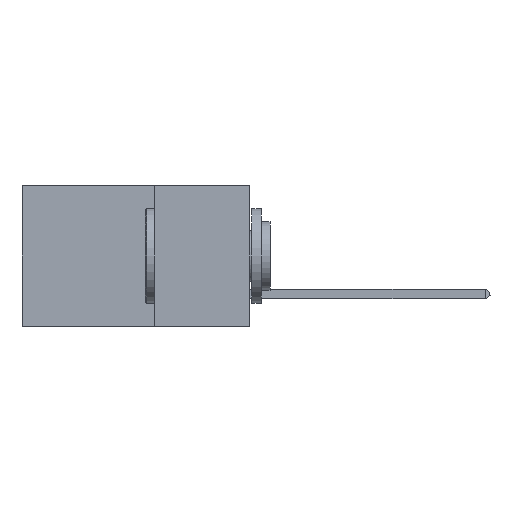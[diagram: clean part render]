
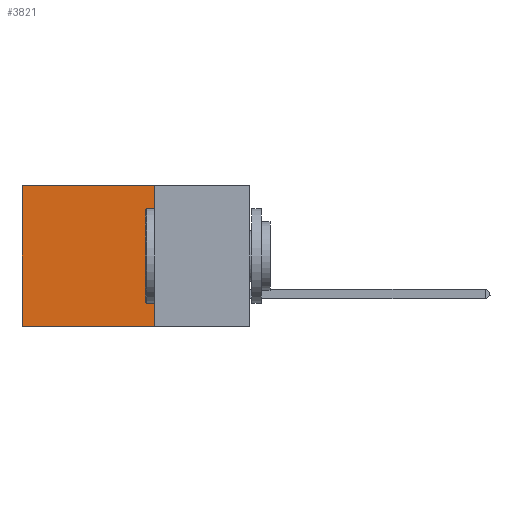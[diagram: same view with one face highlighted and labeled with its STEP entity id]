
A CAD part, left-side view. The second image highlights one B-rep face of the part: STEP entity #3821.
In plain terms, the highlighted planar face has unit normal (-1, 0, 0).
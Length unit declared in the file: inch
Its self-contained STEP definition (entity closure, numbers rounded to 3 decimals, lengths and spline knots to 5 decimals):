
#472 = CARTESIAN_POINT ( 'NONE',  ( 0.2875, 0.25, 0. ) ) ;
#618 = CARTESIAN_POINT ( 'NONE',  ( 0.2875, 0.6, -0.37 ) ) ;
#3821 = ADVANCED_FACE ( 'NONE', ( #30161 ), #40266, .F. ) ;
#4129 = LINE ( 'NONE', #29241, #27058 ) ;
#5090 = EDGE_LOOP ( 'NONE', ( #18821, #26132, #16756, #10674 ) ) ;
#5831 = CARTESIAN_POINT ( 'NONE',  ( 0.2875, 0.25, 0. ) ) ;
#8003 = LINE ( 'NONE', #39644, #36180 ) ;
#9676 = CARTESIAN_POINT ( 'NONE',  ( 0.2875, 0.25, 0. ) ) ;
#10134 = CARTESIAN_POINT ( 'NONE',  ( 0.2875, 0.25, 0. ) ) ;
#10674 = ORIENTED_EDGE ( 'NONE', *, *, #26300, .T. ) ;
#10934 = VERTEX_POINT ( 'NONE', #19697 ) ;
#12505 = EDGE_CURVE ( 'NONE', #19059, #10934, #37296, .T. ) ;
#12753 = EDGE_CURVE ( 'NONE', #10934, #43360, #8003, .T. ) ;
#14618 = EDGE_CURVE ( 'NONE', #18828, #43360, #4129, .T. ) ;
#16756 = ORIENTED_EDGE ( 'NONE', *, *, #12505, .F. ) ;
#18821 = ORIENTED_EDGE ( 'NONE', *, *, #14618, .T. ) ;
#18828 = VERTEX_POINT ( 'NONE', #38321 ) ;
#19059 = VERTEX_POINT ( 'NONE', #5831 ) ;
#19697 = CARTESIAN_POINT ( 'NONE',  ( 0.2875, 0.25, -0.37 ) ) ;
#22315 = AXIS2_PLACEMENT_3D ( 'NONE', #9676, #33602, #33467 ) ;
#23944 = DIRECTION ( 'NONE',  ( 0., 0., -1. ) ) ;
#26132 = ORIENTED_EDGE ( 'NONE', *, *, #12753, .F. ) ;
#26300 = EDGE_CURVE ( 'NONE', #19059, #18828, #30044, .T. ) ;
#27002 = DIRECTION ( 'NONE',  ( 0., 0., -1. ) ) ;
#27058 = VECTOR ( 'NONE', #27002, 39.37008 ) ;
#28961 = VECTOR ( 'NONE', #42107, 39.37008 ) ;
#29241 = CARTESIAN_POINT ( 'NONE',  ( 0.2875, 0.6, 0. ) ) ;
#29252 = DIRECTION ( 'NONE',  ( 0., 1., 0. ) ) ;
#30044 = LINE ( 'NONE', #472, #28961 ) ;
#30161 = FACE_OUTER_BOUND ( 'NONE', #5090, .T. ) ;
#33467 = DIRECTION ( 'NONE',  ( 0., 0., -1. ) ) ;
#33602 = DIRECTION ( 'NONE',  ( 1., 0., 0. ) ) ;
#36180 = VECTOR ( 'NONE', #29252, 39.37008 ) ;
#37296 = LINE ( 'NONE', #10134, #38304 ) ;
#38304 = VECTOR ( 'NONE', #23944, 39.37008 ) ;
#38321 = CARTESIAN_POINT ( 'NONE',  ( 0.2875, 0.6, 0. ) ) ;
#39644 = CARTESIAN_POINT ( 'NONE',  ( 0.2875, 0.25, -0.37 ) ) ;
#40266 = PLANE ( 'NONE',  #22315 ) ;
#42107 = DIRECTION ( 'NONE',  ( 0., 1., 0. ) ) ;
#43360 = VERTEX_POINT ( 'NONE', #618 ) ;
